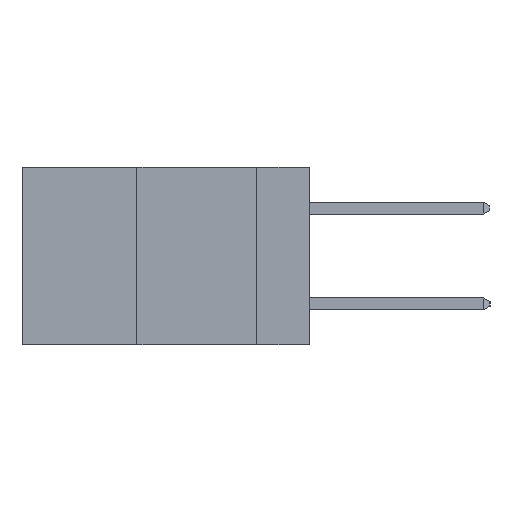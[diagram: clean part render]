
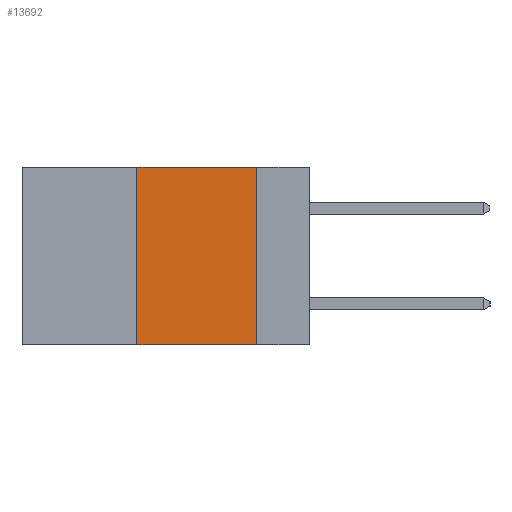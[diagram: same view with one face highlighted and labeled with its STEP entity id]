
A CAD part, left-side view. The second image highlights one B-rep face of the part: STEP entity #13692.
In plain terms, the highlighted planar face has unit normal (-1, 0, 0).
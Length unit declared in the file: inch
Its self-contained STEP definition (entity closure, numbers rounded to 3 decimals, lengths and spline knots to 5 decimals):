
#109 = VERTEX_POINT ( 'NONE', #1011 ) ;
#140 = VERTEX_POINT ( 'NONE', #10683 ) ;
#1011 = CARTESIAN_POINT ( 'NONE',  ( 0., 0.36, -0.37 ) ) ;
#1362 = VECTOR ( 'NONE', #11083, 39.37008 ) ;
#1429 = CARTESIAN_POINT ( 'NONE',  ( 0., 0.11, 0. ) ) ;
#1998 = EDGE_CURVE ( 'NONE', #8517, #6179, #2789, .T. ) ;
#2311 = CARTESIAN_POINT ( 'NONE',  ( 0., 0.6, 0. ) ) ;
#2754 = CARTESIAN_POINT ( 'NONE',  ( 0., 0.6, 0. ) ) ;
#2756 = DIRECTION ( 'NONE',  ( 0., -1., 0. ) ) ;
#2789 = LINE ( 'NONE', #2311, #7016 ) ;
#2799 = PLANE ( 'NONE',  #6370 ) ;
#4174 = CARTESIAN_POINT ( 'NONE',  ( 0., 0.11, 0. ) ) ;
#4386 = LINE ( 'NONE', #4174, #1362 ) ;
#5021 = CARTESIAN_POINT ( 'NONE',  ( 0., 0.36, 0. ) ) ;
#5112 = ORIENTED_EDGE ( 'NONE', *, *, #1998, .F. ) ;
#5787 = EDGE_CURVE ( 'NONE', #6179, #140, #4386, .T. ) ;
#6179 = VERTEX_POINT ( 'NONE', #1429 ) ;
#6370 = AXIS2_PLACEMENT_3D ( 'NONE', #2754, #9520, #10708 ) ;
#6371 = DIRECTION ( 'NONE',  ( 0., 0., 1. ) ) ;
#7016 = VECTOR ( 'NONE', #2756, 39.37008 ) ;
#7418 = VECTOR ( 'NONE', #13826, 39.37008 ) ;
#7578 = ORIENTED_EDGE ( 'NONE', *, *, #8390, .F. ) ;
#8390 = EDGE_CURVE ( 'NONE', #109, #8517, #13070, .T. ) ;
#8517 = VERTEX_POINT ( 'NONE', #9345 ) ;
#9345 = CARTESIAN_POINT ( 'NONE',  ( 0., 0.36, 0. ) ) ;
#9520 = DIRECTION ( 'NONE',  ( 1., 0., 0. ) ) ;
#9978 = EDGE_LOOP ( 'NONE', ( #11720, #5112, #7578, #12492 ) ) ;
#10238 = CARTESIAN_POINT ( 'NONE',  ( 0., 0.6, -0.37 ) ) ;
#10683 = CARTESIAN_POINT ( 'NONE',  ( 0., 0.11, -0.37 ) ) ;
#10708 = DIRECTION ( 'NONE',  ( 0., 0., -1. ) ) ;
#10874 = FACE_OUTER_BOUND ( 'NONE', #9978, .T. ) ;
#11083 = DIRECTION ( 'NONE',  ( 0., 0., -1. ) ) ;
#11720 = ORIENTED_EDGE ( 'NONE', *, *, #5787, .F. ) ;
#12352 = VECTOR ( 'NONE', #6371, 39.37008 ) ;
#12464 = LINE ( 'NONE', #10238, #7418 ) ;
#12492 = ORIENTED_EDGE ( 'NONE', *, *, #12615, .T. ) ;
#12615 = EDGE_CURVE ( 'NONE', #109, #140, #12464, .T. ) ;
#13070 = LINE ( 'NONE', #5021, #12352 ) ;
#13692 = ADVANCED_FACE ( 'NONE', ( #10874 ), #2799, .F. ) ;
#13826 = DIRECTION ( 'NONE',  ( 0., -1., 0. ) ) ;
